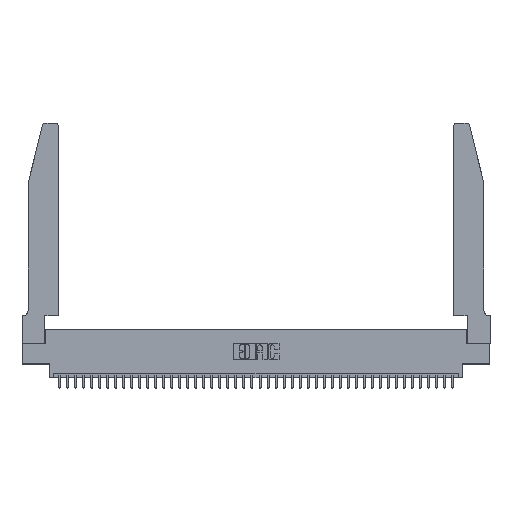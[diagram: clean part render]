
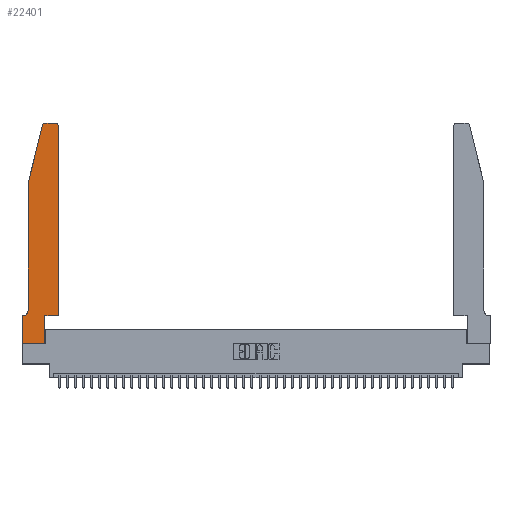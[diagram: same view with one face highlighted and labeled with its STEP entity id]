
A CAD part, top view. The second image highlights one B-rep face of the part: STEP entity #22401.
In plain terms, the highlighted planar face has unit normal (0, 0, 1).
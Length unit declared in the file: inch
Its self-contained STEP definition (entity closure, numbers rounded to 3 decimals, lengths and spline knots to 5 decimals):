
#1190 = EDGE_CURVE ( 'NONE', #12827, #7142, #23932, .T. ) ;
#1353 = ORIENTED_EDGE ( 'NONE', *, *, #1190, .T. ) ;
#1406 = DIRECTION ( 'NONE',  ( 0., 0., 1. ) ) ;
#1763 = VERTEX_POINT ( 'NONE', #33093 ) ;
#2049 = EDGE_CURVE ( 'NONE', #38971, #27491, #27522, .T. ) ;
#2080 = CARTESIAN_POINT ( 'NONE',  ( 0.2865, 0.35, 0.37 ) ) ;
#2412 = AXIS2_PLACEMENT_3D ( 'NONE', #18437, #41439, #21769 ) ;
#3072 = ORIENTED_EDGE ( 'NONE', *, *, #2049, .T. ) ;
#3097 = ORIENTED_EDGE ( 'NONE', *, *, #21627, .T. ) ;
#3960 = CARTESIAN_POINT ( 'NONE',  ( 0.4505, 0.35, 0.37 ) ) ;
#4268 = CIRCLE ( 'NONE', #16696, 0.03 ) ;
#5110 = CARTESIAN_POINT ( 'NONE',  ( 0.0755, 2., 0.37 ) ) ;
#5328 = CARTESIAN_POINT ( 'NONE',  ( 0.284, 2.75, 0.37 ) ) ;
#5919 = EDGE_LOOP ( 'NONE', ( #3072, #38483, #24182, #16610, #1353, #15632, #42210, #20106, #3097, #10950, #20912, #34255 ) ) ;
#6610 = CARTESIAN_POINT ( 'NONE',  ( 0.0755, 2., 0.37 ) ) ;
#6815 = VECTOR ( 'NONE', #36928, 39.37008 ) ;
#7142 = VERTEX_POINT ( 'NONE', #37531 ) ;
#7371 = VECTOR ( 'NONE', #31218, 39.37008 ) ;
#8083 = CARTESIAN_POINT ( 'NONE',  ( 0., 0.35, 0.37 ) ) ;
#8944 = CARTESIAN_POINT ( 'NONE',  ( 0.2605, 2.75, 0.37 ) ) ;
#8952 = DIRECTION ( 'NONE',  ( -1., 0., 0. ) ) ;
#9106 = CIRCLE ( 'NONE', #2412, 0.03 ) ;
#9366 = CARTESIAN_POINT ( 'NONE',  ( 0., 0.35, 0.37 ) ) ;
#9558 = LINE ( 'NONE', #6610, #27196 ) ;
#10950 = ORIENTED_EDGE ( 'NONE', *, *, #18335, .T. ) ;
#11682 = VERTEX_POINT ( 'NONE', #17028 ) ;
#11918 = EDGE_CURVE ( 'NONE', #24952, #37974, #14097, .T. ) ;
#11998 = EDGE_CURVE ( 'NONE', #7142, #13784, #28547, .T. ) ;
#12760 = DIRECTION ( 'NONE',  ( 1., 0., 0. ) ) ;
#12827 = VERTEX_POINT ( 'NONE', #19307 ) ;
#13397 = CARTESIAN_POINT ( 'NONE',  ( 0.0055, 0.42, 0.37 ) ) ;
#13784 = VERTEX_POINT ( 'NONE', #8083 ) ;
#14097 = LINE ( 'NONE', #5110, #30605 ) ;
#14203 = LINE ( 'NONE', #18163, #7371 ) ;
#15632 = ORIENTED_EDGE ( 'NONE', *, *, #11998, .T. ) ;
#15668 = CARTESIAN_POINT ( 'NONE',  ( 0.25487, 2.72718, 0.37 ) ) ;
#16196 = CARTESIAN_POINT ( 'NONE',  ( 0.4205, 2.75, 0.37 ) ) ;
#16610 = ORIENTED_EDGE ( 'NONE', *, *, #26487, .T. ) ;
#16696 = AXIS2_PLACEMENT_3D ( 'NONE', #21551, #1406, #24831 ) ;
#16744 = DIRECTION ( 'NONE',  ( -1., 0., 0. ) ) ;
#17028 = CARTESIAN_POINT ( 'NONE',  ( 0., 0., 0.37 ) ) ;
#17148 = EDGE_CURVE ( 'NONE', #20952, #1763, #25141, .T. ) ;
#17671 = DIRECTION ( 'NONE',  ( 0., -1., 0. ) ) ;
#18163 = CARTESIAN_POINT ( 'NONE',  ( 0., 0., 0.37 ) ) ;
#18335 = EDGE_CURVE ( 'NONE', #37387, #20952, #32222, .T. ) ;
#18437 = CARTESIAN_POINT ( 'NONE',  ( 0.4205, 2.72, 0.37 ) ) ;
#18771 = CARTESIAN_POINT ( 'NONE',  ( 0.0755, 0.35, 0.37 ) ) ;
#18793 = VECTOR ( 'NONE', #38728, 39.37008 ) ;
#19307 = CARTESIAN_POINT ( 'NONE',  ( 0.0755, 0.42, 0.37 ) ) ;
#20106 = ORIENTED_EDGE ( 'NONE', *, *, #24792, .T. ) ;
#20695 = FACE_OUTER_BOUND ( 'NONE', #5919, .T. ) ;
#20912 = ORIENTED_EDGE ( 'NONE', *, *, #17148, .T. ) ;
#20952 = VERTEX_POINT ( 'NONE', #22465 ) ;
#21551 = CARTESIAN_POINT ( 'NONE',  ( 0.284, 2.72, 0.37 ) ) ;
#21627 = EDGE_CURVE ( 'NONE', #31206, #37387, #41843, .T. ) ;
#21769 = DIRECTION ( 'NONE',  ( 1., 0., 0. ) ) ;
#22274 = CARTESIAN_POINT ( 'NONE',  ( 0.2865, 0.35, 0.37 ) ) ;
#22401 = ADVANCED_FACE ( 'NONE', ( #20695 ), #29231, .T. ) ;
#22465 = CARTESIAN_POINT ( 'NONE',  ( 0.4505, 0.35, 0.37 ) ) ;
#23542 = AXIS2_PLACEMENT_3D ( 'NONE', #9366, #32513, #12760 ) ;
#23932 = CIRCLE ( 'NONE', #36148, 0.07 ) ;
#24182 = ORIENTED_EDGE ( 'NONE', *, *, #11918, .T. ) ;
#24333 = VECTOR ( 'NONE', #41962, 39.37008 ) ;
#24792 = EDGE_CURVE ( 'NONE', #11682, #31206, #14203, .T. ) ;
#24831 = DIRECTION ( 'NONE',  ( 1., 0., 0. ) ) ;
#24952 = VERTEX_POINT ( 'NONE', #15668 ) ;
#25141 = LINE ( 'NONE', #3960, #42680 ) ;
#26183 = EDGE_CURVE ( 'NONE', #27491, #24952, #4268, .T. ) ;
#26487 = EDGE_CURVE ( 'NONE', #37974, #12827, #9558, .T. ) ;
#26541 = DIRECTION ( 'NONE',  ( 0., -1., 0. ) ) ;
#27196 = VECTOR ( 'NONE', #26541, 39.37008 ) ;
#27291 = DIRECTION ( 'NONE',  ( 0., 1., 0. ) ) ;
#27491 = VERTEX_POINT ( 'NONE', #5328 ) ;
#27522 = LINE ( 'NONE', #8944, #18793 ) ;
#27937 = CARTESIAN_POINT ( 'NONE',  ( 0.0755, 2., 0.37 ) ) ;
#28389 = DIRECTION ( 'NONE',  ( -0.239, -0.971, 0. ) ) ;
#28547 = LINE ( 'NONE', #18771, #36242 ) ;
#29231 = PLANE ( 'NONE',  #23542 ) ;
#30100 = EDGE_CURVE ( 'NONE', #13784, #11682, #34562, .T. ) ;
#30399 = CARTESIAN_POINT ( 'NONE',  ( 0.2865, 0., 0.37 ) ) ;
#30605 = VECTOR ( 'NONE', #28389, 39.37008 ) ;
#30756 = CARTESIAN_POINT ( 'NONE',  ( 0., 0., 0.37 ) ) ;
#31206 = VERTEX_POINT ( 'NONE', #30399 ) ;
#31218 = DIRECTION ( 'NONE',  ( 1., 0., 0. ) ) ;
#31890 = EDGE_CURVE ( 'NONE', #1763, #38971, #9106, .T. ) ;
#32222 = LINE ( 'NONE', #33611, #6815 ) ;
#32513 = DIRECTION ( 'NONE',  ( 0., 0., 1. ) ) ;
#33093 = CARTESIAN_POINT ( 'NONE',  ( 0.4505, 2.72, 0.37 ) ) ;
#33611 = CARTESIAN_POINT ( 'NONE',  ( 0.4505, 0.35, 0.37 ) ) ;
#34255 = ORIENTED_EDGE ( 'NONE', *, *, #31890, .T. ) ;
#34562 = LINE ( 'NONE', #30756, #42341 ) ;
#36148 = AXIS2_PLACEMENT_3D ( 'NONE', #13397, #36431, #16744 ) ;
#36242 = VECTOR ( 'NONE', #8952, 39.37008 ) ;
#36431 = DIRECTION ( 'NONE',  ( 0., 0., -1. ) ) ;
#36928 = DIRECTION ( 'NONE',  ( 1., 0., 0. ) ) ;
#37387 = VERTEX_POINT ( 'NONE', #2080 ) ;
#37531 = CARTESIAN_POINT ( 'NONE',  ( 0.0055, 0.35, 0.37 ) ) ;
#37974 = VERTEX_POINT ( 'NONE', #27937 ) ;
#38483 = ORIENTED_EDGE ( 'NONE', *, *, #26183, .T. ) ;
#38728 = DIRECTION ( 'NONE',  ( -1., 0., 0. ) ) ;
#38971 = VERTEX_POINT ( 'NONE', #16196 ) ;
#41439 = DIRECTION ( 'NONE',  ( 0., 0., 1. ) ) ;
#41843 = LINE ( 'NONE', #22274, #24333 ) ;
#41962 = DIRECTION ( 'NONE',  ( 0., 1., 0. ) ) ;
#42210 = ORIENTED_EDGE ( 'NONE', *, *, #30100, .T. ) ;
#42341 = VECTOR ( 'NONE', #17671, 39.37008 ) ;
#42680 = VECTOR ( 'NONE', #27291, 39.37008 ) ;
